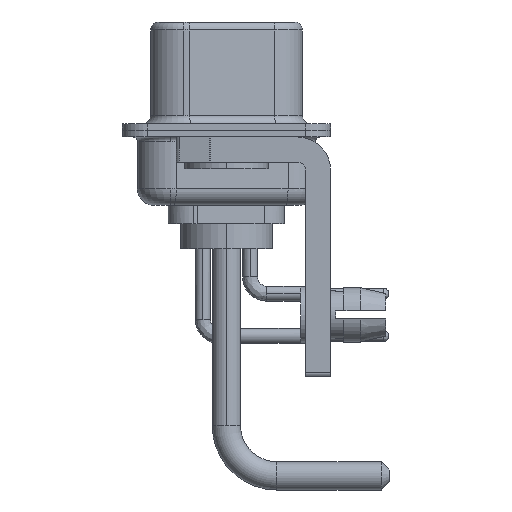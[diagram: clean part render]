
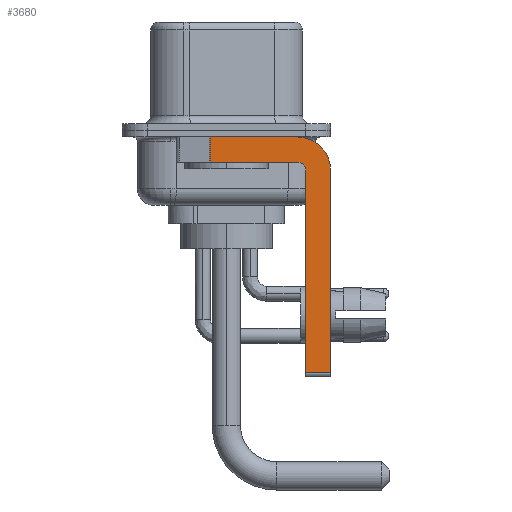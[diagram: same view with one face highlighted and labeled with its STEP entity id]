
A CAD part, left-side view. The second image highlights one B-rep face of the part: STEP entity #3680.
In plain terms, the highlighted planar face has unit normal (-1, 0, 0).
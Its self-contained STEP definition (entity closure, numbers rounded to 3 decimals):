
#32 = VERTEX_POINT ( 'NONE', #21589 ) ;
#170 = LINE ( 'NONE', #21004, #9068 ) ;
#461 = EDGE_CURVE ( 'NONE', #17337, #18887, #170, .T. ) ;
#831 = VERTEX_POINT ( 'NONE', #25647 ) ;
#1442 = ORIENTED_EDGE ( 'NONE', *, *, #22779, .F. ) ;
#1598 = DIRECTION ( 'NONE',  ( 0., 0., 1. ) ) ;
#1781 = VERTEX_POINT ( 'NONE', #2504 ) ;
#2504 = CARTESIAN_POINT ( 'NONE',  ( -2.9, -4.75, -2.4 ) ) ;
#2640 = EDGE_CURVE ( 'NONE', #12837, #18887, #6392, .T. ) ;
#3146 = DIRECTION ( 'NONE',  ( 1., 0., 0. ) ) ;
#3680 = ADVANCED_FACE ( 'NONE', ( #13687 ), #9298, .F. ) ;
#4292 = VECTOR ( 'NONE', #4514, 1000. ) ;
#4514 = DIRECTION ( 'NONE',  ( 0., -1., 0. ) ) ;
#4687 = CARTESIAN_POINT ( 'NONE',  ( -2.9, -6.25, -2.4 ) ) ;
#4934 = CARTESIAN_POINT ( 'NONE',  ( -2.9, -4.25, -2.4 ) ) ;
#5645 = DIRECTION ( 'NONE',  ( 0., 0., -1. ) ) ;
#6392 = LINE ( 'NONE', #14764, #26433 ) ;
#6396 = CARTESIAN_POINT ( 'NONE',  ( -2.9, -4.25, -1.9 ) ) ;
#6410 = LINE ( 'NONE', #12591, #4292 ) ;
#6662 = DIRECTION ( 'NONE',  ( 0., -1., 0. ) ) ;
#7600 = DIRECTION ( 'NONE',  ( -1., 0., 0. ) ) ;
#8416 = EDGE_CURVE ( 'NONE', #24675, #32, #6410, .T. ) ;
#8484 = EDGE_CURVE ( 'NONE', #12837, #1781, #11198, .T. ) ;
#9068 = VECTOR ( 'NONE', #21142, 1000. ) ;
#9298 = PLANE ( 'NONE',  #25661 ) ;
#10510 = ORIENTED_EDGE ( 'NONE', *, *, #18981, .T. ) ;
#10800 = ORIENTED_EDGE ( 'NONE', *, *, #22585, .F. ) ;
#11198 = LINE ( 'NONE', #23712, #13912 ) ;
#11586 = AXIS2_PLACEMENT_3D ( 'NONE', #21640, #25891, #25754 ) ;
#11663 = CARTESIAN_POINT ( 'NONE',  ( -2.9, 0.978, -1.9 ) ) ;
#11830 = ORIENTED_EDGE ( 'NONE', *, *, #8484, .F. ) ;
#12591 = CARTESIAN_POINT ( 'NONE',  ( -2.9, 3., -0.4 ) ) ;
#12837 = VERTEX_POINT ( 'NONE', #19506 ) ;
#13687 = FACE_OUTER_BOUND ( 'NONE', #17007, .T. ) ;
#13833 = VERTEX_POINT ( 'NONE', #16456 ) ;
#13878 = LINE ( 'NONE', #11663, #15023 ) ;
#13912 = VECTOR ( 'NONE', #22035, 1000. ) ;
#14242 = CIRCLE ( 'NONE', #11586, 2. ) ;
#14741 = EDGE_CURVE ( 'NONE', #13833, #831, #22740, .T. ) ;
#14764 = CARTESIAN_POINT ( 'NONE',  ( -2.9, -4.25, -14.55 ) ) ;
#15023 = VECTOR ( 'NONE', #5645, 1000. ) ;
#15132 = CARTESIAN_POINT ( 'NONE',  ( -2.9, -6.25, -14.55 ) ) ;
#15467 = ORIENTED_EDGE ( 'NONE', *, *, #2640, .T. ) ;
#16456 = CARTESIAN_POINT ( 'NONE',  ( -2.9, -4.25, -1.9 ) ) ;
#17007 = EDGE_LOOP ( 'NONE', ( #17748, #10510, #26454, #1442, #11830, #15467, #19103, #10800 ) ) ;
#17337 = VERTEX_POINT ( 'NONE', #4687 ) ;
#17748 = ORIENTED_EDGE ( 'NONE', *, *, #8416, .F. ) ;
#18887 = VERTEX_POINT ( 'NONE', #15132 ) ;
#18981 = EDGE_CURVE ( 'NONE', #24675, #831, #13878, .T. ) ;
#19103 = ORIENTED_EDGE ( 'NONE', *, *, #461, .F. ) ;
#19506 = CARTESIAN_POINT ( 'NONE',  ( -2.9, -4.75, -14.55 ) ) ;
#21004 = CARTESIAN_POINT ( 'NONE',  ( -2.9, -6.25, -2.4 ) ) ;
#21142 = DIRECTION ( 'NONE',  ( 0., 0., -1. ) ) ;
#21589 = CARTESIAN_POINT ( 'NONE',  ( -2.9, -4.25, -0.4 ) ) ;
#21640 = CARTESIAN_POINT ( 'NONE',  ( -2.9, -4.25, -2.4 ) ) ;
#22035 = DIRECTION ( 'NONE',  ( 0., 0., 1. ) ) ;
#22044 = CARTESIAN_POINT ( 'NONE',  ( -2.9, 0.978, -0.4 ) ) ;
#22123 = CIRCLE ( 'NONE', #24769, 0.5 ) ;
#22473 = DIRECTION ( 'NONE',  ( 0., 1., 0. ) ) ;
#22585 = EDGE_CURVE ( 'NONE', #32, #17337, #14242, .T. ) ;
#22740 = LINE ( 'NONE', #6396, #26709 ) ;
#22779 = EDGE_CURVE ( 'NONE', #1781, #13833, #22123, .T. ) ;
#23712 = CARTESIAN_POINT ( 'NONE',  ( -2.9, -4.75, -14.8 ) ) ;
#24254 = DIRECTION ( 'NONE',  ( 0., 0., -1. ) ) ;
#24675 = VERTEX_POINT ( 'NONE', #22044 ) ;
#24769 = AXIS2_PLACEMENT_3D ( 'NONE', #26424, #7600, #1598 ) ;
#25647 = CARTESIAN_POINT ( 'NONE',  ( -2.9, 0.978, -1.9 ) ) ;
#25661 = AXIS2_PLACEMENT_3D ( 'NONE', #4934, #3146, #24254 ) ;
#25754 = DIRECTION ( 'NONE',  ( 0., 0., -1. ) ) ;
#25891 = DIRECTION ( 'NONE',  ( 1., 0., 0. ) ) ;
#26424 = CARTESIAN_POINT ( 'NONE',  ( -2.9, -4.25, -2.4 ) ) ;
#26433 = VECTOR ( 'NONE', #6662, 1000. ) ;
#26454 = ORIENTED_EDGE ( 'NONE', *, *, #14741, .F. ) ;
#26709 = VECTOR ( 'NONE', #22473, 1000. ) ;
